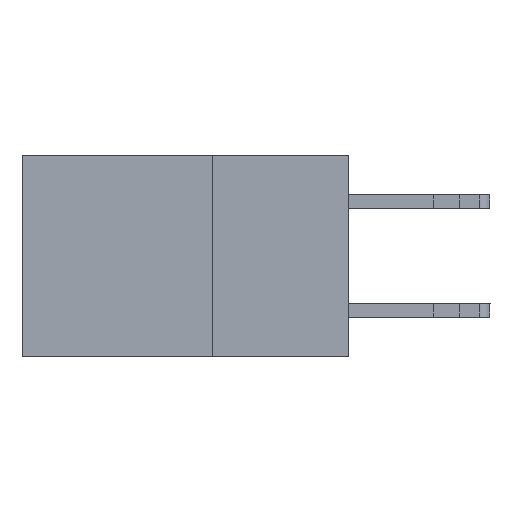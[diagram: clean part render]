
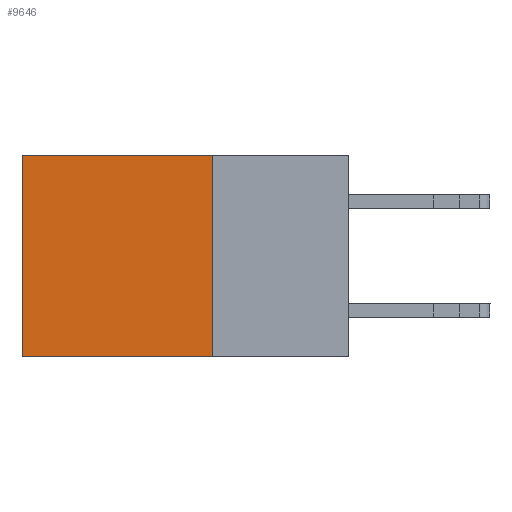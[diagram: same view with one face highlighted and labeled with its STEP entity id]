
A CAD part, left-side view. The second image highlights one B-rep face of the part: STEP entity #9646.
In plain terms, the highlighted planar face has unit normal (-1, 0, 0).
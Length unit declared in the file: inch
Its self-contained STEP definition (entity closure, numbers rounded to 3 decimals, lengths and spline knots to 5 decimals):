
#393 = CARTESIAN_POINT ( 'NONE',  ( 0.2615, 0.25, 0. ) ) ;
#675 = CARTESIAN_POINT ( 'NONE',  ( 0.2615, 0.25, -0.37 ) ) ;
#1812 = DIRECTION ( 'NONE',  ( 0., 1., 0. ) ) ;
#1838 = VECTOR ( 'NONE', #2205, 39.37008 ) ;
#1902 = ORIENTED_EDGE ( 'NONE', *, *, #12433, .F. ) ;
#2205 = DIRECTION ( 'NONE',  ( 0., 0., -1. ) ) ;
#2264 = VECTOR ( 'NONE', #5075, 39.37008 ) ;
#3024 = CARTESIAN_POINT ( 'NONE',  ( 0.2615, 0.25, 0. ) ) ;
#4193 = VECTOR ( 'NONE', #1812, 39.37008 ) ;
#4422 = ORIENTED_EDGE ( 'NONE', *, *, #12245, .T. ) ;
#5075 = DIRECTION ( 'NONE',  ( 0., 1., 0. ) ) ;
#6964 = CARTESIAN_POINT ( 'NONE',  ( 0.2615, 0.6, 0. ) ) ;
#7353 = VERTEX_POINT ( 'NONE', #6964 ) ;
#7660 = LINE ( 'NONE', #3024, #4193 ) ;
#8067 = DIRECTION ( 'NONE',  ( 1., 0., 0. ) ) ;
#8085 = PLANE ( 'NONE',  #13467 ) ;
#9052 = LINE ( 'NONE', #14724, #2264 ) ;
#9593 = CARTESIAN_POINT ( 'NONE',  ( 0.2615, 0.6, -0.37 ) ) ;
#9646 = ADVANCED_FACE ( 'NONE', ( #13498 ), #8085, .F. ) ;
#9791 = CARTESIAN_POINT ( 'NONE',  ( 0.2615, 0.25, -0.37 ) ) ;
#9983 = ORIENTED_EDGE ( 'NONE', *, *, #14667, .T. ) ;
#10478 = ORIENTED_EDGE ( 'NONE', *, *, #14541, .F. ) ;
#10561 = DIRECTION ( 'NONE',  ( 0., 0., -1. ) ) ;
#11016 = VERTEX_POINT ( 'NONE', #9593 ) ;
#12245 = EDGE_CURVE ( 'NONE', #13521, #7353, #7660, .T. ) ;
#12334 = VERTEX_POINT ( 'NONE', #675 ) ;
#12433 = EDGE_CURVE ( 'NONE', #13521, #12334, #14470, .T. ) ;
#12977 = CARTESIAN_POINT ( 'NONE',  ( 0.2615, 0.25, -0.37 ) ) ;
#13099 = LINE ( 'NONE', #13804, #15683 ) ;
#13467 = AXIS2_PLACEMENT_3D ( 'NONE', #12977, #8067, #10561 ) ;
#13498 = FACE_OUTER_BOUND ( 'NONE', #14428, .T. ) ;
#13521 = VERTEX_POINT ( 'NONE', #393 ) ;
#13752 = DIRECTION ( 'NONE',  ( 0., 0., -1. ) ) ;
#13804 = CARTESIAN_POINT ( 'NONE',  ( 0.2615, 0.6, -0.37 ) ) ;
#14428 = EDGE_LOOP ( 'NONE', ( #9983, #10478, #1902, #4422 ) ) ;
#14470 = LINE ( 'NONE', #9791, #1838 ) ;
#14541 = EDGE_CURVE ( 'NONE', #12334, #11016, #9052, .T. ) ;
#14667 = EDGE_CURVE ( 'NONE', #7353, #11016, #13099, .T. ) ;
#14724 = CARTESIAN_POINT ( 'NONE',  ( 0.2615, 0.25, -0.37 ) ) ;
#15683 = VECTOR ( 'NONE', #13752, 39.37008 ) ;
